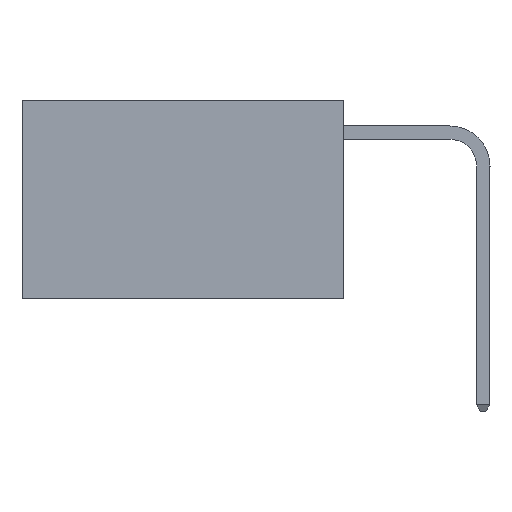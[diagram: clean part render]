
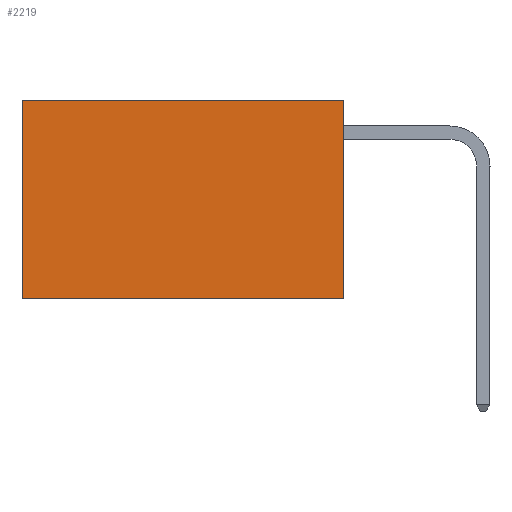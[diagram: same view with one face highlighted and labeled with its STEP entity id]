
A CAD part, left-side view. The second image highlights one B-rep face of the part: STEP entity #2219.
In plain terms, the highlighted planar face has unit normal (-1, 0, 0).
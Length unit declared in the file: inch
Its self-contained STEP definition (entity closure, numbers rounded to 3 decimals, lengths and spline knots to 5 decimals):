
#86 = CARTESIAN_POINT ( 'NONE',  ( 0.2625, 0., 0. ) ) ;
#720 = FACE_OUTER_BOUND ( 'NONE', #9443, .T. ) ;
#798 = CARTESIAN_POINT ( 'NONE',  ( 0.2625, 0., 0. ) ) ;
#799 = CARTESIAN_POINT ( 'NONE',  ( 0.2625, 0., 0. ) ) ;
#2219 = ADVANCED_FACE ( 'NONE', ( #720 ), #7080, .F. ) ;
#2340 = VERTEX_POINT ( 'NONE', #86 ) ;
#2474 = AXIS2_PLACEMENT_3D ( 'NONE', #798, #6548, #9728 ) ;
#2513 = DIRECTION ( 'NONE',  ( 0., 0., -1. ) ) ;
#2711 = VECTOR ( 'NONE', #8787, 39.37008 ) ;
#2731 = CARTESIAN_POINT ( 'NONE',  ( 0.2625, 0., -0.37 ) ) ;
#3528 = CARTESIAN_POINT ( 'NONE',  ( 0.2625, 0., 0. ) ) ;
#4017 = CARTESIAN_POINT ( 'NONE',  ( 0.2625, 0., -0.37 ) ) ;
#4116 = CARTESIAN_POINT ( 'NONE',  ( 0.2625, 0.6, 0. ) ) ;
#4660 = VECTOR ( 'NONE', #5980, 39.37008 ) ;
#4888 = EDGE_CURVE ( 'NONE', #7376, #10148, #7195, .T. ) ;
#5474 = EDGE_CURVE ( 'NONE', #2340, #7376, #6736, .T. ) ;
#5757 = CARTESIAN_POINT ( 'NONE',  ( 0.2625, 0.6, -0.37 ) ) ;
#5980 = DIRECTION ( 'NONE',  ( 0., 0., -1. ) ) ;
#6473 = VECTOR ( 'NONE', #2513, 39.37008 ) ;
#6548 = DIRECTION ( 'NONE',  ( 1., 0., 0. ) ) ;
#6612 = ORIENTED_EDGE ( 'NONE', *, *, #5474, .T. ) ;
#6736 = LINE ( 'NONE', #799, #11295 ) ;
#6803 = LINE ( 'NONE', #3528, #6473 ) ;
#7073 = VERTEX_POINT ( 'NONE', #2731 ) ;
#7078 = CARTESIAN_POINT ( 'NONE',  ( 0.2625, 0.6, 0. ) ) ;
#7080 = PLANE ( 'NONE',  #2474 ) ;
#7195 = LINE ( 'NONE', #4116, #4660 ) ;
#7376 = VERTEX_POINT ( 'NONE', #7078 ) ;
#7695 = DIRECTION ( 'NONE',  ( 0., 1., 0. ) ) ;
#7802 = LINE ( 'NONE', #4017, #2711 ) ;
#8182 = EDGE_CURVE ( 'NONE', #2340, #7073, #6803, .T. ) ;
#8283 = ORIENTED_EDGE ( 'NONE', *, *, #8182, .F. ) ;
#8787 = DIRECTION ( 'NONE',  ( 0., 1., 0. ) ) ;
#9443 = EDGE_LOOP ( 'NONE', ( #10400, #11074, #8283, #6612 ) ) ;
#9728 = DIRECTION ( 'NONE',  ( 0., 0., -1. ) ) ;
#10148 = VERTEX_POINT ( 'NONE', #5757 ) ;
#10400 = ORIENTED_EDGE ( 'NONE', *, *, #4888, .T. ) ;
#11074 = ORIENTED_EDGE ( 'NONE', *, *, #11107, .F. ) ;
#11107 = EDGE_CURVE ( 'NONE', #7073, #10148, #7802, .T. ) ;
#11295 = VECTOR ( 'NONE', #7695, 39.37008 ) ;
